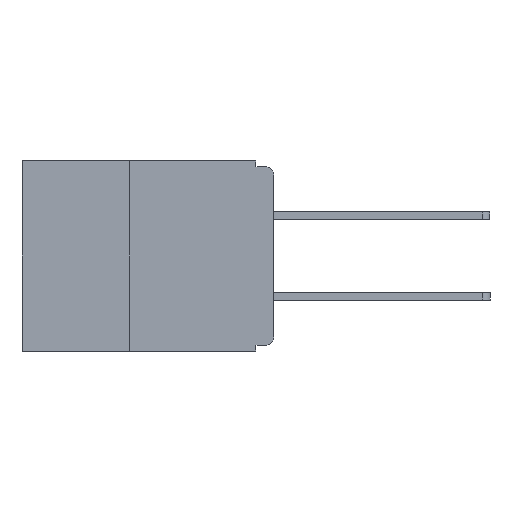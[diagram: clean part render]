
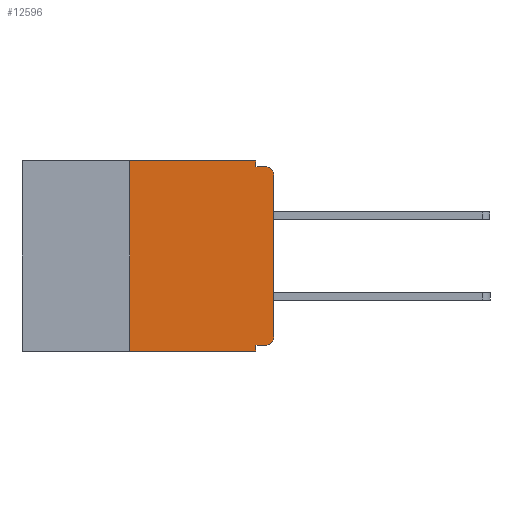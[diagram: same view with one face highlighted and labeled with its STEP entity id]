
A CAD part, left-side view. The second image highlights one B-rep face of the part: STEP entity #12596.
In plain terms, the highlighted planar face has unit normal (-1, 0, 0).
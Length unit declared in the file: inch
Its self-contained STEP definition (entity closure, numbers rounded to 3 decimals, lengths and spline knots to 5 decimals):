
#427 = DIRECTION ( 'NONE',  ( 0., -1., 0. ) ) ;
#450 = CARTESIAN_POINT ( 'NONE',  ( 0., 0.437, 0. ) ) ;
#761 = DIRECTION ( 'NONE',  ( 0., 0., -1. ) ) ;
#788 = CARTESIAN_POINT ( 'NONE',  ( 0., 0.25, 0. ) ) ;
#801 = CARTESIAN_POINT ( 'NONE',  ( 0., 0.015, -0.01 ) ) ;
#822 = DIRECTION ( 'NONE',  ( -1., 0., 0. ) ) ;
#847 = CARTESIAN_POINT ( 'NONE',  ( 0., 0.015, -0.305 ) ) ;
#991 = ORIENTED_EDGE ( 'NONE', *, *, #15905, .F. ) ;
#1131 = VERTEX_POINT ( 'NONE', #5876 ) ;
#1174 = AXIS2_PLACEMENT_3D ( 'NONE', #1688, #11271, #3083 ) ;
#1346 = ORIENTED_EDGE ( 'NONE', *, *, #5526, .F. ) ;
#1361 = DIRECTION ( 'NONE',  ( 0., -1., 0. ) ) ;
#1688 = CARTESIAN_POINT ( 'NONE',  ( 0., 0.015, -0.025 ) ) ;
#1717 = VECTOR ( 'NONE', #11653, 39.37008 ) ;
#1797 = ORIENTED_EDGE ( 'NONE', *, *, #11969, .F. ) ;
#1894 = CARTESIAN_POINT ( 'NONE',  ( 0., 0.25, -0.33 ) ) ;
#1953 = LINE ( 'NONE', #9650, #9231 ) ;
#1972 = LINE ( 'NONE', #16534, #12872 ) ;
#2105 = ORIENTED_EDGE ( 'NONE', *, *, #5511, .T. ) ;
#2374 = CARTESIAN_POINT ( 'NONE',  ( 0., 0.031, 0. ) ) ;
#2934 = CARTESIAN_POINT ( 'NONE',  ( 0., 0.031, -0.01 ) ) ;
#3083 = DIRECTION ( 'NONE',  ( 0., 0., -1. ) ) ;
#3272 = CIRCLE ( 'NONE', #1174, 0.015 ) ;
#3301 = LINE ( 'NONE', #450, #10581 ) ;
#3658 = CARTESIAN_POINT ( 'NONE',  ( 0., 0.015, -0.32 ) ) ;
#3864 = CARTESIAN_POINT ( 'NONE',  ( 0., 0., -0.305 ) ) ;
#3898 = VERTEX_POINT ( 'NONE', #7281 ) ;
#3922 = VECTOR ( 'NONE', #5294, 39.37008 ) ;
#3954 = VERTEX_POINT ( 'NONE', #3864 ) ;
#4135 = ORIENTED_EDGE ( 'NONE', *, *, #14689, .F. ) ;
#4394 = VECTOR ( 'NONE', #1361, 39.37008 ) ;
#4436 = VERTEX_POINT ( 'NONE', #3658 ) ;
#4507 = VERTEX_POINT ( 'NONE', #1894 ) ;
#4914 = CARTESIAN_POINT ( 'NONE',  ( 0., 0.437, -0.33 ) ) ;
#5104 = ORIENTED_EDGE ( 'NONE', *, *, #14644, .T. ) ;
#5177 = EDGE_CURVE ( 'NONE', #4507, #8213, #7396, .T. ) ;
#5274 = CARTESIAN_POINT ( 'NONE',  ( 0., 0., 0. ) ) ;
#5294 = DIRECTION ( 'NONE',  ( 0., 0., 1. ) ) ;
#5465 = ORIENTED_EDGE ( 'NONE', *, *, #15118, .F. ) ;
#5511 = EDGE_CURVE ( 'NONE', #4436, #3954, #6565, .T. ) ;
#5526 = EDGE_CURVE ( 'NONE', #8213, #12581, #3301, .T. ) ;
#5632 = EDGE_CURVE ( 'NONE', #4507, #17003, #9282, .T. ) ;
#5876 = CARTESIAN_POINT ( 'NONE',  ( 0., 0., -0.025 ) ) ;
#6347 = ORIENTED_EDGE ( 'NONE', *, *, #5632, .T. ) ;
#6554 = EDGE_CURVE ( 'NONE', #3954, #1131, #11178, .T. ) ;
#6565 = CIRCLE ( 'NONE', #13140, 0.015 ) ;
#7281 = CARTESIAN_POINT ( 'NONE',  ( 0., 0.031, -0.32 ) ) ;
#7396 = LINE ( 'NONE', #8731, #17053 ) ;
#7478 = VECTOR ( 'NONE', #10621, 39.37008 ) ;
#8125 = CARTESIAN_POINT ( 'NONE',  ( 0., 0.437, 0. ) ) ;
#8213 = VERTEX_POINT ( 'NONE', #788 ) ;
#8295 = AXIS2_PLACEMENT_3D ( 'NONE', #8125, #17282, #9466 ) ;
#8553 = DIRECTION ( 'NONE',  ( 0., 0., 1. ) ) ;
#8649 = DIRECTION ( 'NONE',  ( 0., 1., 0. ) ) ;
#8731 = CARTESIAN_POINT ( 'NONE',  ( 0., 0.25, -0.33 ) ) ;
#9015 = LINE ( 'NONE', #15464, #1717 ) ;
#9187 = CARTESIAN_POINT ( 'NONE',  ( 0., 0.031, -0.33 ) ) ;
#9231 = VECTOR ( 'NONE', #17449, 39.37008 ) ;
#9282 = LINE ( 'NONE', #4914, #4394 ) ;
#9466 = DIRECTION ( 'NONE',  ( 0., 0., -1. ) ) ;
#9650 = CARTESIAN_POINT ( 'NONE',  ( 0., 0., -0.01 ) ) ;
#10239 = EDGE_LOOP ( 'NONE', ( #10345, #5104, #5465, #1797, #1346, #10762, #6347, #991, #4135, #2105 ) ) ;
#10345 = ORIENTED_EDGE ( 'NONE', *, *, #6554, .T. ) ;
#10581 = VECTOR ( 'NONE', #427, 39.37008 ) ;
#10621 = DIRECTION ( 'NONE',  ( 0., 0., -1. ) ) ;
#10762 = ORIENTED_EDGE ( 'NONE', *, *, #5177, .F. ) ;
#11075 = LINE ( 'NONE', #2374, #7478 ) ;
#11178 = LINE ( 'NONE', #5274, #3922 ) ;
#11271 = DIRECTION ( 'NONE',  ( -1., 0., 0. ) ) ;
#11653 = DIRECTION ( 'NONE',  ( 0., 0., -1. ) ) ;
#11687 = FACE_OUTER_BOUND ( 'NONE', #10239, .T. ) ;
#11969 = EDGE_CURVE ( 'NONE', #12581, #15676, #11075, .T. ) ;
#12581 = VERTEX_POINT ( 'NONE', #13512 ) ;
#12596 = ADVANCED_FACE ( 'NONE', ( #11687 ), #16030, .F. ) ;
#12872 = VECTOR ( 'NONE', #8649, 39.37008 ) ;
#13140 = AXIS2_PLACEMENT_3D ( 'NONE', #847, #822, #761 ) ;
#13512 = CARTESIAN_POINT ( 'NONE',  ( 0., 0.031, 0. ) ) ;
#14644 = EDGE_CURVE ( 'NONE', #1131, #14896, #3272, .T. ) ;
#14689 = EDGE_CURVE ( 'NONE', #4436, #3898, #1972, .T. ) ;
#14896 = VERTEX_POINT ( 'NONE', #801 ) ;
#15118 = EDGE_CURVE ( 'NONE', #15676, #14896, #1953, .T. ) ;
#15464 = CARTESIAN_POINT ( 'NONE',  ( 0., 0.031, -0.33 ) ) ;
#15676 = VERTEX_POINT ( 'NONE', #2934 ) ;
#15905 = EDGE_CURVE ( 'NONE', #3898, #17003, #9015, .T. ) ;
#16030 = PLANE ( 'NONE',  #8295 ) ;
#16534 = CARTESIAN_POINT ( 'NONE',  ( 0., 0., -0.32 ) ) ;
#17003 = VERTEX_POINT ( 'NONE', #9187 ) ;
#17053 = VECTOR ( 'NONE', #8553, 39.37008 ) ;
#17282 = DIRECTION ( 'NONE',  ( 1., 0., 0. ) ) ;
#17449 = DIRECTION ( 'NONE',  ( 0., -1., 0. ) ) ;
